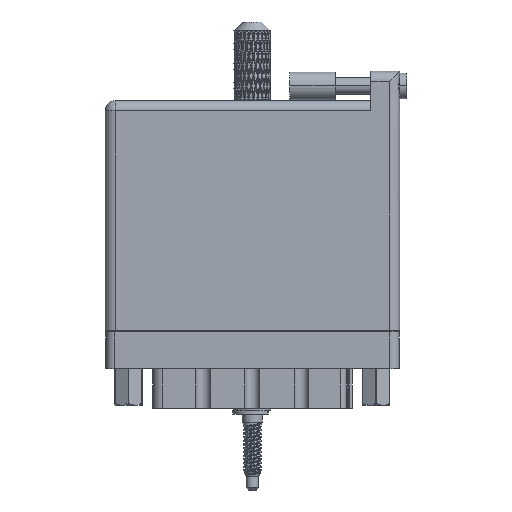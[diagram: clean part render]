
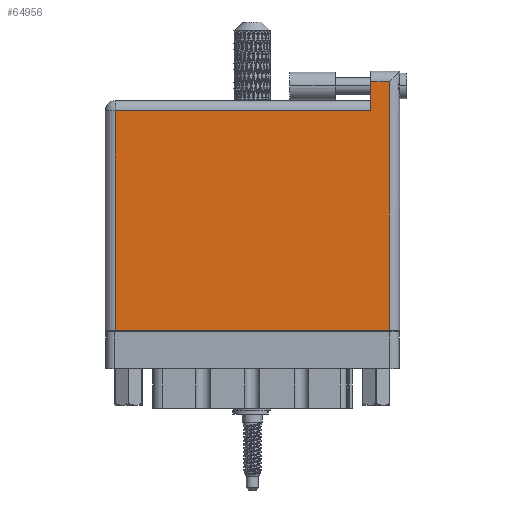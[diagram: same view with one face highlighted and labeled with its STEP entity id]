
A CAD part, front view. The second image highlights one B-rep face of the part: STEP entity #64956.
In plain terms, the highlighted face is planar.
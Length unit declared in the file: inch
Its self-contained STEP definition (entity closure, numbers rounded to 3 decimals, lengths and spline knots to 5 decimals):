
#1980 = VECTOR ( 'NONE', #5884, 39.37008 ) ;
#5884 = DIRECTION ( 'NONE',  ( -1., 0., 0. ) ) ;
#6325 = VERTEX_POINT ( 'NONE', #41496 ) ;
#8054 = EDGE_CURVE ( 'NONE', #6325, #42147, #81612, .T. ) ;
#9098 = EDGE_CURVE ( 'NONE', #42147, #89789, #11625, .T. ) ;
#9504 = FACE_OUTER_BOUND ( 'NONE', #65796, .T. ) ;
#11625 = LINE ( 'NONE', #62397, #29776 ) ;
#11842 = EDGE_CURVE ( 'NONE', #19576, #63408, #43445, .T. ) ;
#17761 = CARTESIAN_POINT ( 'NONE',  ( 0., 0., 0. ) ) ;
#18319 = CARTESIAN_POINT ( 'NONE',  ( 1.811, 1.696, 0. ) ) ;
#18773 = CARTESIAN_POINT ( 'NONE',  ( 1.938, 1.766, 0. ) ) ;
#18937 = ORIENTED_EDGE ( 'NONE', *, *, #105746, .T. ) ;
#19005 = PLANE ( 'NONE',  #54251 ) ;
#19576 = VERTEX_POINT ( 'NONE', #22953 ) ;
#22953 = CARTESIAN_POINT ( 'NONE',  ( 1.938, 1.696, 0. ) ) ;
#25113 = VECTOR ( 'NONE', #64163, 39.37008 ) ;
#26474 = ORIENTED_EDGE ( 'NONE', *, *, #88066, .T. ) ;
#28221 = CARTESIAN_POINT ( 'NONE',  ( 0., 1.696, 0. ) ) ;
#29295 = LINE ( 'NONE', #18773, #25113 ) ;
#29776 = VECTOR ( 'NONE', #44747, 39.37008 ) ;
#33411 = ORIENTED_EDGE ( 'NONE', *, *, #11842, .T. ) ;
#33584 = CARTESIAN_POINT ( 'NONE',  ( 0.07, 0., 0. ) ) ;
#37214 = DIRECTION ( 'NONE',  ( -1., 0., 0. ) ) ;
#41496 = CARTESIAN_POINT ( 'NONE',  ( 1.811, 1.496, 0. ) ) ;
#42147 = VERTEX_POINT ( 'NONE', #68508 ) ;
#43445 = LINE ( 'NONE', #28221, #53238 ) ;
#44747 = DIRECTION ( 'NONE',  ( 0., -1., 0. ) ) ;
#46782 = EDGE_CURVE ( 'NONE', #75279, #19576, #29295, .T. ) ;
#48215 = CARTESIAN_POINT ( 'NONE',  ( 1.811, 1.766, 0. ) ) ;
#53238 = VECTOR ( 'NONE', #37214, 39.37008 ) ;
#54251 = AXIS2_PLACEMENT_3D ( 'NONE', #111033, #57765, #108331 ) ;
#57478 = ORIENTED_EDGE ( 'NONE', *, *, #8054, .T. ) ;
#57765 = DIRECTION ( 'NONE',  ( 0., 0., -1. ) ) ;
#62374 = VECTOR ( 'NONE', #101967, 39.37008 ) ;
#62397 = CARTESIAN_POINT ( 'NONE',  ( 0.07, 0., 0. ) ) ;
#63408 = VERTEX_POINT ( 'NONE', #18319 ) ;
#64163 = DIRECTION ( 'NONE',  ( 0., 1., 0. ) ) ;
#64956 = ADVANCED_FACE ( 'NONE', ( #9504 ), #19005, .F. ) ;
#65796 = EDGE_LOOP ( 'NONE', ( #26474, #108509, #33411, #18937, #57478, #115718 ) ) ;
#67697 = CARTESIAN_POINT ( 'NONE',  ( 1.938, 0., 0. ) ) ;
#68508 = CARTESIAN_POINT ( 'NONE',  ( 0.07, 1.496, 0. ) ) ;
#70498 = DIRECTION ( 'NONE',  ( 1., 0., 0. ) ) ;
#75279 = VERTEX_POINT ( 'NONE', #67697 ) ;
#81612 = LINE ( 'NONE', #112727, #1980 ) ;
#83368 = VECTOR ( 'NONE', #70498, 39.37008 ) ;
#84700 = LINE ( 'NONE', #17761, #83368 ) ;
#88066 = EDGE_CURVE ( 'NONE', #89789, #75279, #84700, .T. ) ;
#89789 = VERTEX_POINT ( 'NONE', #33584 ) ;
#98521 = LINE ( 'NONE', #48215, #62374 ) ;
#101967 = DIRECTION ( 'NONE',  ( 0., -1., 0. ) ) ;
#105746 = EDGE_CURVE ( 'NONE', #63408, #6325, #98521, .T. ) ;
#108331 = DIRECTION ( 'NONE',  ( -1., 0., 0. ) ) ;
#108509 = ORIENTED_EDGE ( 'NONE', *, *, #46782, .T. ) ;
#111033 = CARTESIAN_POINT ( 'NONE',  ( 0., 1.566, 0. ) ) ;
#112727 = CARTESIAN_POINT ( 'NONE',  ( 0., 1.496, 0. ) ) ;
#115718 = ORIENTED_EDGE ( 'NONE', *, *, #9098, .T. ) ;
